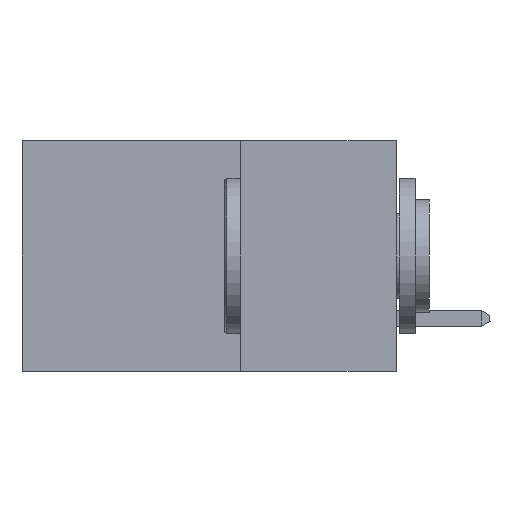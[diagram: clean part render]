
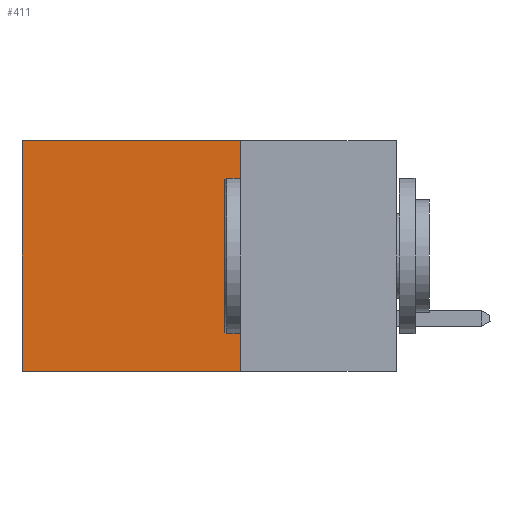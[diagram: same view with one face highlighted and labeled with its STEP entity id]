
A CAD part, left-side view. The second image highlights one B-rep face of the part: STEP entity #411.
In plain terms, the highlighted planar face has unit normal (-1, 0, 0).
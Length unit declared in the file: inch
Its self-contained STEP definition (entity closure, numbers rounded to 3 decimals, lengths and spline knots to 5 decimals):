
#41 = VERTEX_POINT ( 'NONE', #10127 ) ;
#131 = VECTOR ( 'NONE', #8265, 39.37008 ) ;
#177 = ORIENTED_EDGE ( 'NONE', *, *, #1447, .F. ) ;
#411 = ADVANCED_FACE ( 'NONE', ( #2705 ), #13817, .F. ) ;
#549 = AXIS2_PLACEMENT_3D ( 'NONE', #2657, #12066, #7962 ) ;
#1223 = DIRECTION ( 'NONE',  ( 0., 1., 0. ) ) ;
#1447 = EDGE_CURVE ( 'NONE', #10931, #41, #8212, .T. ) ;
#1927 = CARTESIAN_POINT ( 'NONE',  ( 0.298, 0.25, -0.37 ) ) ;
#2657 = CARTESIAN_POINT ( 'NONE',  ( 0.298, 0.25, 0. ) ) ;
#2705 = FACE_OUTER_BOUND ( 'NONE', #13440, .T. ) ;
#4227 = CARTESIAN_POINT ( 'NONE',  ( 0.298, 0.25, 0. ) ) ;
#4294 = DIRECTION ( 'NONE',  ( 0., 0., -1. ) ) ;
#5326 = DIRECTION ( 'NONE',  ( 0., 0., -1. ) ) ;
#6411 = LINE ( 'NONE', #9661, #11344 ) ;
#6629 = ORIENTED_EDGE ( 'NONE', *, *, #6884, .T. ) ;
#6780 = CARTESIAN_POINT ( 'NONE',  ( 0.298, 0.25, 0. ) ) ;
#6884 = EDGE_CURVE ( 'NONE', #13335, #7982, #11512, .T. ) ;
#7133 = EDGE_CURVE ( 'NONE', #7982, #41, #6411, .T. ) ;
#7962 = DIRECTION ( 'NONE',  ( 0., 0., -1. ) ) ;
#7982 = VERTEX_POINT ( 'NONE', #9574 ) ;
#8212 = LINE ( 'NONE', #13241, #13700 ) ;
#8265 = DIRECTION ( 'NONE',  ( 0., 1., 0. ) ) ;
#8444 = ORIENTED_EDGE ( 'NONE', *, *, #9379, .F. ) ;
#9379 = EDGE_CURVE ( 'NONE', #13335, #10931, #10967, .T. ) ;
#9574 = CARTESIAN_POINT ( 'NONE',  ( 0.298, 0.6, 0. ) ) ;
#9661 = CARTESIAN_POINT ( 'NONE',  ( 0.298, 0.6, 0. ) ) ;
#9981 = ORIENTED_EDGE ( 'NONE', *, *, #7133, .T. ) ;
#10127 = CARTESIAN_POINT ( 'NONE',  ( 0.298, 0.6, -0.37 ) ) ;
#10365 = CARTESIAN_POINT ( 'NONE',  ( 0.298, 0.25, 0. ) ) ;
#10931 = VERTEX_POINT ( 'NONE', #1927 ) ;
#10967 = LINE ( 'NONE', #4227, #13684 ) ;
#11344 = VECTOR ( 'NONE', #4294, 39.37008 ) ;
#11512 = LINE ( 'NONE', #10365, #131 ) ;
#12066 = DIRECTION ( 'NONE',  ( 1., 0., 0. ) ) ;
#13241 = CARTESIAN_POINT ( 'NONE',  ( 0.298, 0.25, -0.37 ) ) ;
#13335 = VERTEX_POINT ( 'NONE', #6780 ) ;
#13440 = EDGE_LOOP ( 'NONE', ( #9981, #177, #8444, #6629 ) ) ;
#13684 = VECTOR ( 'NONE', #5326, 39.37008 ) ;
#13700 = VECTOR ( 'NONE', #1223, 39.37008 ) ;
#13817 = PLANE ( 'NONE',  #549 ) ;
